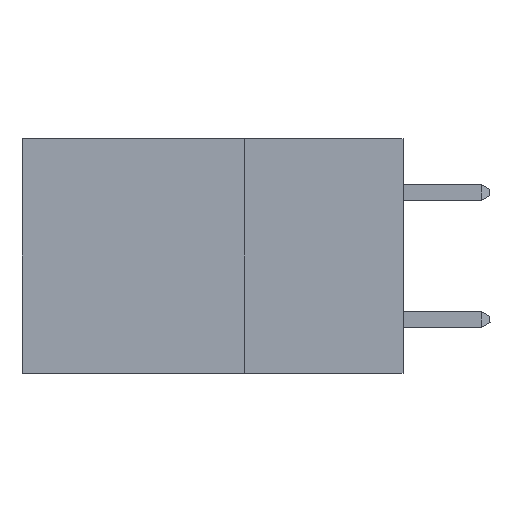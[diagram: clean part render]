
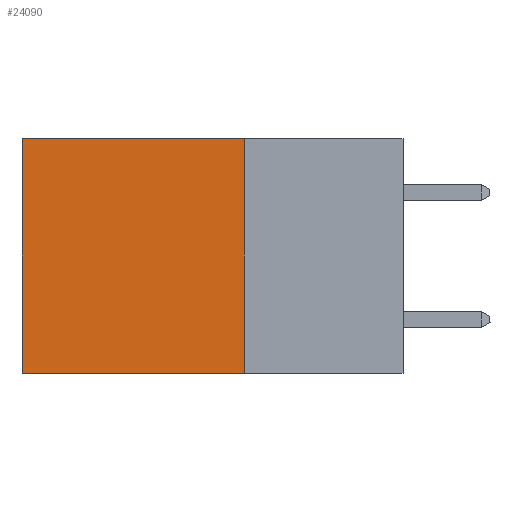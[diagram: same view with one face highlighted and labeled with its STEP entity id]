
A CAD part, left-side view. The second image highlights one B-rep face of the part: STEP entity #24090.
In plain terms, the highlighted planar face has unit normal (-1, 0, 0).
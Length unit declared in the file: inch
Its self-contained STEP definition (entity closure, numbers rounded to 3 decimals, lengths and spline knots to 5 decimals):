
#590 = PLANE ( 'NONE',  #16433 ) ;
#1075 = CARTESIAN_POINT ( 'NONE',  ( 0.2875, 0.6, 0. ) ) ;
#1267 = CARTESIAN_POINT ( 'NONE',  ( 0.2875, 0.25, 0. ) ) ;
#1643 = ORIENTED_EDGE ( 'NONE', *, *, #14732, .F. ) ;
#3690 = VECTOR ( 'NONE', #15071, 39.37008 ) ;
#5677 = CARTESIAN_POINT ( 'NONE',  ( 0.2875, 0.25, 0. ) ) ;
#5735 = VERTEX_POINT ( 'NONE', #33269 ) ;
#6664 = LINE ( 'NONE', #1075, #30372 ) ;
#6851 = CARTESIAN_POINT ( 'NONE',  ( 0.2875, 0.6, 0. ) ) ;
#7680 = VECTOR ( 'NONE', #11585, 39.37008 ) ;
#8897 = LINE ( 'NONE', #1267, #7680 ) ;
#9741 = EDGE_CURVE ( 'NONE', #10276, #29083, #8897, .T. ) ;
#10276 = VERTEX_POINT ( 'NONE', #19663 ) ;
#11585 = DIRECTION ( 'NONE',  ( 0., 1., 0. ) ) ;
#11737 = VERTEX_POINT ( 'NONE', #12722 ) ;
#11825 = DIRECTION ( 'NONE',  ( 0., 1., 0. ) ) ;
#12621 = ORIENTED_EDGE ( 'NONE', *, *, #19764, .T. ) ;
#12722 = CARTESIAN_POINT ( 'NONE',  ( 0.2875, 0.6, -0.37 ) ) ;
#14732 = EDGE_CURVE ( 'NONE', #10276, #5735, #25259, .T. ) ;
#15071 = DIRECTION ( 'NONE',  ( 0., 0., -1. ) ) ;
#16433 = AXIS2_PLACEMENT_3D ( 'NONE', #5677, #25991, #23447 ) ;
#19105 = CARTESIAN_POINT ( 'NONE',  ( 0.2875, 0.25, -0.37 ) ) ;
#19663 = CARTESIAN_POINT ( 'NONE',  ( 0.2875, 0.25, 0. ) ) ;
#19764 = EDGE_CURVE ( 'NONE', #29083, #11737, #6664, .T. ) ;
#21988 = EDGE_CURVE ( 'NONE', #5735, #11737, #27240, .T. ) ;
#22827 = EDGE_LOOP ( 'NONE', ( #12621, #28184, #1643, #29564 ) ) ;
#23447 = DIRECTION ( 'NONE',  ( 0., 0., -1. ) ) ;
#24090 = ADVANCED_FACE ( 'NONE', ( #28364 ), #590, .F. ) ;
#24546 = VECTOR ( 'NONE', #11825, 39.37008 ) ;
#25087 = CARTESIAN_POINT ( 'NONE',  ( 0.2875, 0.25, 0. ) ) ;
#25259 = LINE ( 'NONE', #25087, #3690 ) ;
#25991 = DIRECTION ( 'NONE',  ( 1., 0., 0. ) ) ;
#27240 = LINE ( 'NONE', #19105, #24546 ) ;
#28184 = ORIENTED_EDGE ( 'NONE', *, *, #21988, .F. ) ;
#28364 = FACE_OUTER_BOUND ( 'NONE', #22827, .T. ) ;
#29083 = VERTEX_POINT ( 'NONE', #6851 ) ;
#29564 = ORIENTED_EDGE ( 'NONE', *, *, #9741, .T. ) ;
#30372 = VECTOR ( 'NONE', #32550, 39.37008 ) ;
#32550 = DIRECTION ( 'NONE',  ( 0., 0., -1. ) ) ;
#33269 = CARTESIAN_POINT ( 'NONE',  ( 0.2875, 0.25, -0.37 ) ) ;
